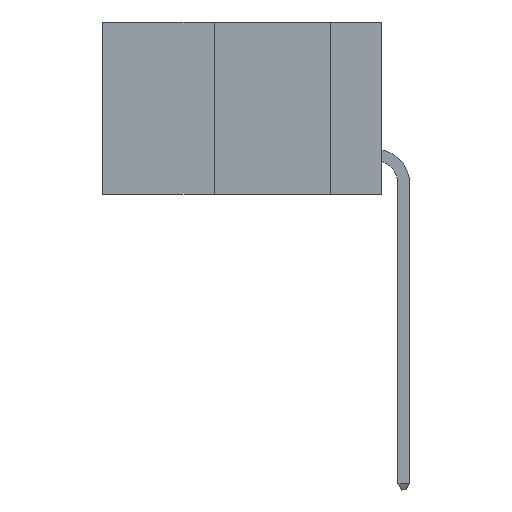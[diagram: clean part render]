
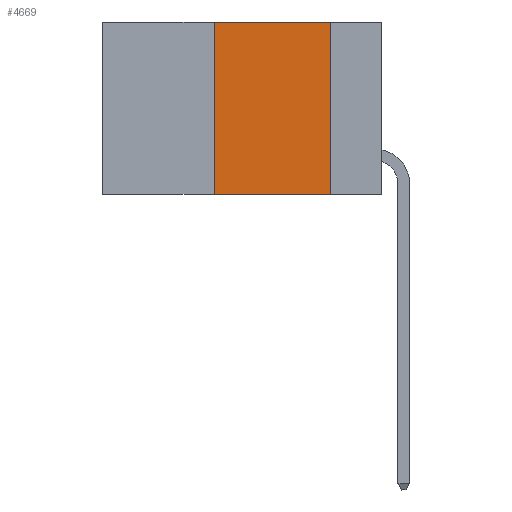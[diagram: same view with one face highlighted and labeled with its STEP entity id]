
A CAD part, left-side view. The second image highlights one B-rep face of the part: STEP entity #4669.
In plain terms, the highlighted planar face has unit normal (-1, 0, 0).
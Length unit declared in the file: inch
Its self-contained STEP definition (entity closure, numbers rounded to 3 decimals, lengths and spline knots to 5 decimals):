
#85 = LINE ( 'NONE', #2075, #7943 ) ;
#111 = EDGE_CURVE ( 'NONE', #1545, #12854, #3529, .T. ) ;
#838 = VECTOR ( 'NONE', #7399, 39.37008 ) ;
#1545 = VERTEX_POINT ( 'NONE', #8448 ) ;
#2075 = CARTESIAN_POINT ( 'NONE',  ( 0., 0.11, 0. ) ) ;
#2135 = CARTESIAN_POINT ( 'NONE',  ( 0., 0.11, 0. ) ) ;
#2582 = DIRECTION ( 'NONE',  ( 0., -1., 0. ) ) ;
#2802 = CARTESIAN_POINT ( 'NONE',  ( 0., 0.11, -0.37 ) ) ;
#3272 = CARTESIAN_POINT ( 'NONE',  ( 0., 0.6, -0.37 ) ) ;
#3529 = LINE ( 'NONE', #3272, #838 ) ;
#3690 = CARTESIAN_POINT ( 'NONE',  ( 0., 0.6, 0. ) ) ;
#3955 = EDGE_CURVE ( 'NONE', #1545, #10291, #7036, .T. ) ;
#4029 = VECTOR ( 'NONE', #2582, 39.37008 ) ;
#4223 = VECTOR ( 'NONE', #6226, 39.37008 ) ;
#4421 = EDGE_CURVE ( 'NONE', #10291, #8044, #6189, .T. ) ;
#4669 = ADVANCED_FACE ( 'NONE', ( #11735 ), #9329, .F. ) ;
#6189 = LINE ( 'NONE', #3690, #4029 ) ;
#6223 = ORIENTED_EDGE ( 'NONE', *, *, #4421, .F. ) ;
#6226 = DIRECTION ( 'NONE',  ( 0., 0., 1. ) ) ;
#7036 = LINE ( 'NONE', #8325, #4223 ) ;
#7395 = EDGE_CURVE ( 'NONE', #8044, #12854, #85, .T. ) ;
#7399 = DIRECTION ( 'NONE',  ( 0., -1., 0. ) ) ;
#7765 = AXIS2_PLACEMENT_3D ( 'NONE', #12598, #12503, #11459 ) ;
#7943 = VECTOR ( 'NONE', #12680, 39.37008 ) ;
#8044 = VERTEX_POINT ( 'NONE', #2135 ) ;
#8325 = CARTESIAN_POINT ( 'NONE',  ( 0., 0.36, 0. ) ) ;
#8448 = CARTESIAN_POINT ( 'NONE',  ( 0., 0.36, -0.37 ) ) ;
#9329 = PLANE ( 'NONE',  #7765 ) ;
#9776 = CARTESIAN_POINT ( 'NONE',  ( 0., 0.36, 0. ) ) ;
#10291 = VERTEX_POINT ( 'NONE', #9776 ) ;
#11459 = DIRECTION ( 'NONE',  ( 0., 0., -1. ) ) ;
#11696 = ORIENTED_EDGE ( 'NONE', *, *, #3955, .F. ) ;
#11735 = FACE_OUTER_BOUND ( 'NONE', #12274, .T. ) ;
#12274 = EDGE_LOOP ( 'NONE', ( #12315, #6223, #11696, #13361 ) ) ;
#12315 = ORIENTED_EDGE ( 'NONE', *, *, #7395, .F. ) ;
#12503 = DIRECTION ( 'NONE',  ( 1., 0., 0. ) ) ;
#12598 = CARTESIAN_POINT ( 'NONE',  ( 0., 0.6, 0. ) ) ;
#12680 = DIRECTION ( 'NONE',  ( 0., 0., -1. ) ) ;
#12854 = VERTEX_POINT ( 'NONE', #2802 ) ;
#13361 = ORIENTED_EDGE ( 'NONE', *, *, #111, .T. ) ;
